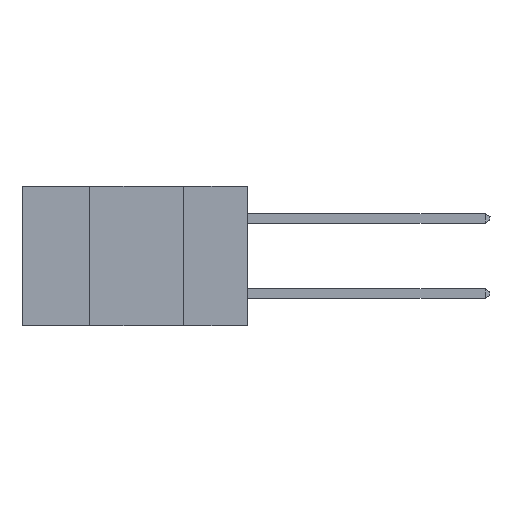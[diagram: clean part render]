
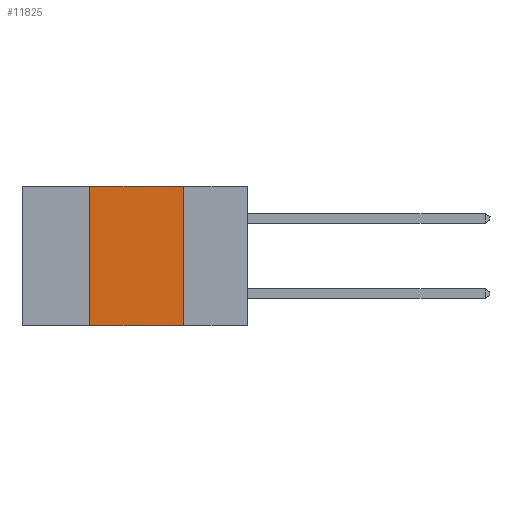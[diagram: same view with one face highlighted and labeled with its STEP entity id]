
A CAD part, left-side view. The second image highlights one B-rep face of the part: STEP entity #11825.
In plain terms, the highlighted planar face has unit normal (-1, 0, 0).
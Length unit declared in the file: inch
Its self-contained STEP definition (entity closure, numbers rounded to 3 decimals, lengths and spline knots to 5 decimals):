
#596 = VECTOR ( 'NONE', #2738, 39.37008 ) ;
#793 = LINE ( 'NONE', #18981, #2229 ) ;
#1199 = CARTESIAN_POINT ( 'NONE',  ( 0., 0.17, 0. ) ) ;
#1335 = VECTOR ( 'NONE', #10478, 39.37008 ) ;
#1839 = VERTEX_POINT ( 'NONE', #9444 ) ;
#1933 = VERTEX_POINT ( 'NONE', #4971 ) ;
#2229 = VECTOR ( 'NONE', #10311, 39.37008 ) ;
#2436 = ORIENTED_EDGE ( 'NONE', *, *, #17113, .F. ) ;
#2451 = FACE_OUTER_BOUND ( 'NONE', #5739, .T. ) ;
#2602 = DIRECTION ( 'NONE',  ( 1., 0., 0. ) ) ;
#2738 = DIRECTION ( 'NONE',  ( 0., 0., 1. ) ) ;
#3464 = EDGE_CURVE ( 'NONE', #1933, #17917, #12792, .T. ) ;
#4133 = PLANE ( 'NONE',  #16707 ) ;
#4971 = CARTESIAN_POINT ( 'NONE',  ( 0., 0.42, 0. ) ) ;
#5198 = EDGE_CURVE ( 'NONE', #17917, #6165, #793, .T. ) ;
#5739 = EDGE_LOOP ( 'NONE', ( #14642, #17642, #2436, #13985 ) ) ;
#6165 = VERTEX_POINT ( 'NONE', #14376 ) ;
#7698 = VECTOR ( 'NONE', #10979, 39.37008 ) ;
#8898 = LINE ( 'NONE', #14617, #596 ) ;
#8944 = CARTESIAN_POINT ( 'NONE',  ( 0., 0.6, 0. ) ) ;
#9444 = CARTESIAN_POINT ( 'NONE',  ( 0., 0.42, -0.37 ) ) ;
#10311 = DIRECTION ( 'NONE',  ( 0., 0., -1. ) ) ;
#10313 = LINE ( 'NONE', #12342, #7698 ) ;
#10432 = CARTESIAN_POINT ( 'NONE',  ( 0., 0.6, 0. ) ) ;
#10478 = DIRECTION ( 'NONE',  ( 0., -1., 0. ) ) ;
#10979 = DIRECTION ( 'NONE',  ( 0., -1., 0. ) ) ;
#11791 = DIRECTION ( 'NONE',  ( 0., 0., -1. ) ) ;
#11825 = ADVANCED_FACE ( 'NONE', ( #2451 ), #4133, .F. ) ;
#12342 = CARTESIAN_POINT ( 'NONE',  ( 0., 0.6, -0.37 ) ) ;
#12792 = LINE ( 'NONE', #8944, #1335 ) ;
#13985 = ORIENTED_EDGE ( 'NONE', *, *, #17521, .T. ) ;
#14376 = CARTESIAN_POINT ( 'NONE',  ( 0., 0.17, -0.37 ) ) ;
#14617 = CARTESIAN_POINT ( 'NONE',  ( 0., 0.42, 0. ) ) ;
#14642 = ORIENTED_EDGE ( 'NONE', *, *, #5198, .F. ) ;
#16707 = AXIS2_PLACEMENT_3D ( 'NONE', #10432, #2602, #11791 ) ;
#17113 = EDGE_CURVE ( 'NONE', #1839, #1933, #8898, .T. ) ;
#17521 = EDGE_CURVE ( 'NONE', #1839, #6165, #10313, .T. ) ;
#17642 = ORIENTED_EDGE ( 'NONE', *, *, #3464, .F. ) ;
#17917 = VERTEX_POINT ( 'NONE', #1199 ) ;
#18981 = CARTESIAN_POINT ( 'NONE',  ( 0., 0.17, 0. ) ) ;
